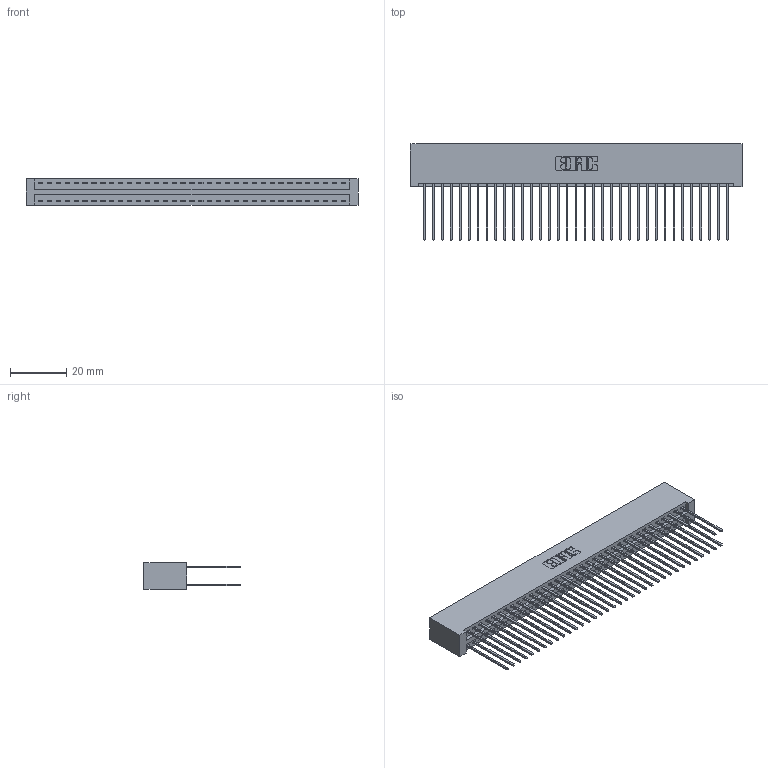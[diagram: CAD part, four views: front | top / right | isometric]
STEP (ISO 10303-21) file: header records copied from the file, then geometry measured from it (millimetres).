
FILE_DESCRIPTION (( 'STEP AP203' ), '1' );
FILE_NAME ('346-070-541-201.STEP', '2022-05-24T21:39:35', ( '' ), ( '' ), 'SwSTEP 2.0', 'SolidWorks 2020', '' );
FILE_SCHEMA (( 'CONFIG_CONTROL_DESIGN' ));
Length unit declared in the file: inch
Products named in the file (3): 345-292-001_345-293-141; 346-070-541-201; 346 Part_No Mounting Lugs
Assembly tree (71 placements, depth 2):
  346-070-541-201
    346 Part_No Mounting Lugs
    345-292-001_345-293-141  x70
Bounding box: 118.36 x 34.29 x 9.4 mm (x, y, z)
Volume: 12462.5 mm3; surface area: 19109.7 mm2
Topology: 71 solids, 71 shells, 3754 faces, 11155 edges, 7342 vertices
Faces by surface type: plane 2522, cylinder 1232
Entity records: 23525 total; most frequent: CARTESIAN_POINT 3884, ORIENTED_EDGE 3818, DIRECTION 3469, EDGE_CURVE 1909, LINE 1645, VECTOR 1645, VERTEX_POINT 1270, AXIS2_PLACEMENT_3D 912
